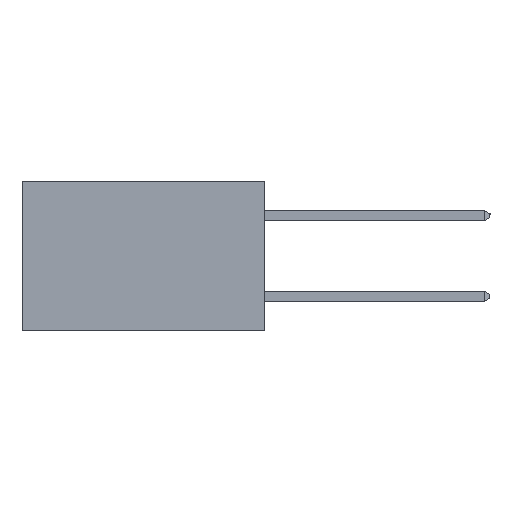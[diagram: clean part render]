
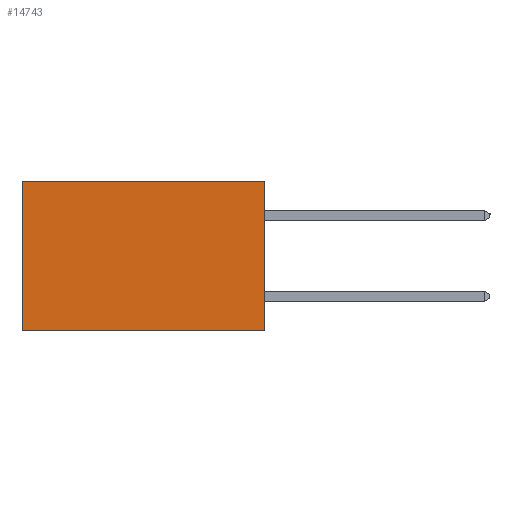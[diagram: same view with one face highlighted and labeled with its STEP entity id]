
A CAD part, left-side view. The second image highlights one B-rep face of the part: STEP entity #14743.
In plain terms, the highlighted planar face has unit normal (-1, 0, 0).
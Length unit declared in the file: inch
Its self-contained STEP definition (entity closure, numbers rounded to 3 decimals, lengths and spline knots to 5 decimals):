
#326 = DIRECTION ( 'NONE',  ( 0., 0., -1. ) ) ;
#1335 = ORIENTED_EDGE ( 'NONE', *, *, #5728, .F. ) ;
#1770 = EDGE_CURVE ( 'NONE', #13892, #2598, #6135, .T. ) ;
#2004 = CARTESIAN_POINT ( 'NONE',  ( 0.2615, 0., -0.37 ) ) ;
#2083 = VERTEX_POINT ( 'NONE', #9303 ) ;
#2598 = VERTEX_POINT ( 'NONE', #3103 ) ;
#3103 = CARTESIAN_POINT ( 'NONE',  ( 0.2615, 0.6, -0.37 ) ) ;
#3753 = CARTESIAN_POINT ( 'NONE',  ( 0.2615, 0., -0.37 ) ) ;
#4078 = LINE ( 'NONE', #6429, #6844 ) ;
#5537 = CARTESIAN_POINT ( 'NONE',  ( 0.2615, 0., -0.37 ) ) ;
#5687 = EDGE_CURVE ( 'NONE', #2083, #14817, #7248, .T. ) ;
#5728 = EDGE_CURVE ( 'NONE', #2083, #13892, #7003, .T. ) ;
#5732 = VECTOR ( 'NONE', #9530, 39.37008 ) ;
#5987 = AXIS2_PLACEMENT_3D ( 'NONE', #5537, #13647, #12460 ) ;
#6135 = LINE ( 'NONE', #8461, #6995 ) ;
#6220 = VECTOR ( 'NONE', #8004, 39.37008 ) ;
#6297 = DIRECTION ( 'NONE',  ( 0., 1., 0. ) ) ;
#6429 = CARTESIAN_POINT ( 'NONE',  ( 0.2615, 0.6, -0.37 ) ) ;
#6844 = VECTOR ( 'NONE', #326, 39.37008 ) ;
#6995 = VECTOR ( 'NONE', #6297, 39.37008 ) ;
#7003 = LINE ( 'NONE', #3753, #6220 ) ;
#7248 = LINE ( 'NONE', #8432, #5732 ) ;
#7942 = EDGE_CURVE ( 'NONE', #14817, #2598, #4078, .T. ) ;
#8004 = DIRECTION ( 'NONE',  ( 0., 0., -1. ) ) ;
#8432 = CARTESIAN_POINT ( 'NONE',  ( 0.2615, 0., 0. ) ) ;
#8461 = CARTESIAN_POINT ( 'NONE',  ( 0.2615, 0., -0.37 ) ) ;
#8943 = PLANE ( 'NONE',  #5987 ) ;
#9303 = CARTESIAN_POINT ( 'NONE',  ( 0.2615, 0., 0. ) ) ;
#9530 = DIRECTION ( 'NONE',  ( 0., 1., 0. ) ) ;
#11360 = FACE_OUTER_BOUND ( 'NONE', #11876, .T. ) ;
#11876 = EDGE_LOOP ( 'NONE', ( #13021, #14071, #1335, #13563 ) ) ;
#12460 = DIRECTION ( 'NONE',  ( 0., 0., -1. ) ) ;
#13021 = ORIENTED_EDGE ( 'NONE', *, *, #7942, .T. ) ;
#13563 = ORIENTED_EDGE ( 'NONE', *, *, #5687, .T. ) ;
#13647 = DIRECTION ( 'NONE',  ( 1., 0., 0. ) ) ;
#13892 = VERTEX_POINT ( 'NONE', #2004 ) ;
#14071 = ORIENTED_EDGE ( 'NONE', *, *, #1770, .F. ) ;
#14743 = ADVANCED_FACE ( 'NONE', ( #11360 ), #8943, .F. ) ;
#14817 = VERTEX_POINT ( 'NONE', #15052 ) ;
#15052 = CARTESIAN_POINT ( 'NONE',  ( 0.2615, 0.6, 0. ) ) ;
